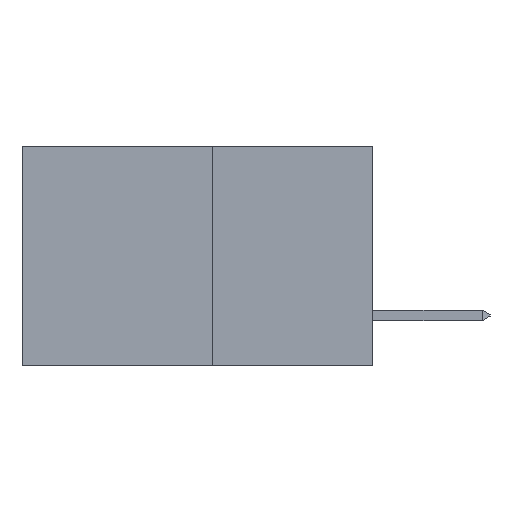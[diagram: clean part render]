
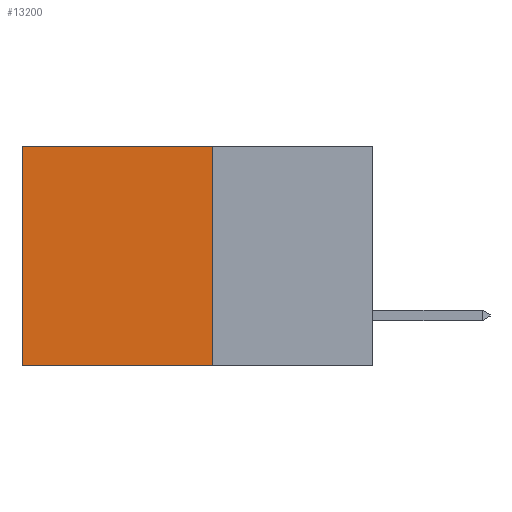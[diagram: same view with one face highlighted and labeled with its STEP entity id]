
A CAD part, left-side view. The second image highlights one B-rep face of the part: STEP entity #13200.
In plain terms, the highlighted planar face has unit normal (-1, 0, 0).
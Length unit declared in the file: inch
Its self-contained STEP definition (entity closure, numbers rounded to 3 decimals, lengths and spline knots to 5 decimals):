
#7 = DIRECTION ( 'NONE',  ( 0., 1., 0. ) ) ;
#88 = ORIENTED_EDGE ( 'NONE', *, *, #18496, .T. ) ;
#1582 = DIRECTION ( 'NONE',  ( 0., 0., -1. ) ) ;
#2198 = DIRECTION ( 'NONE',  ( 0., 0., -1. ) ) ;
#2292 = ORIENTED_EDGE ( 'NONE', *, *, #22013, .T. ) ;
#4181 = VERTEX_POINT ( 'NONE', #13359 ) ;
#4532 = CARTESIAN_POINT ( 'NONE',  ( 0.277, 0.27, -0.37 ) ) ;
#4536 = CARTESIAN_POINT ( 'NONE',  ( 0.277, 0.59, -0.37 ) ) ;
#6033 = LINE ( 'NONE', #4536, #24186 ) ;
#7980 = VECTOR ( 'NONE', #15490, 39.37008 ) ;
#8729 = LINE ( 'NONE', #22567, #7980 ) ;
#9309 = PLANE ( 'NONE',  #23987 ) ;
#9402 = CARTESIAN_POINT ( 'NONE',  ( 0.277, 0.59, -0.37 ) ) ;
#9446 = VERTEX_POINT ( 'NONE', #9402 ) ;
#10930 = ORIENTED_EDGE ( 'NONE', *, *, #21144, .F. ) ;
#13200 = ADVANCED_FACE ( 'NONE', ( #29827 ), #9309, .F. ) ;
#13251 = EDGE_CURVE ( 'NONE', #4181, #9446, #15998, .T. ) ;
#13359 = CARTESIAN_POINT ( 'NONE',  ( 0.277, 0.27, -0.37 ) ) ;
#13468 = VERTEX_POINT ( 'NONE', #26701 ) ;
#14346 = CARTESIAN_POINT ( 'NONE',  ( 0.277, 0.59, 0. ) ) ;
#15490 = DIRECTION ( 'NONE',  ( 0., 1., 0. ) ) ;
#15998 = LINE ( 'NONE', #28307, #21582 ) ;
#16497 = DIRECTION ( 'NONE',  ( 1., 0., 0. ) ) ;
#16927 = DIRECTION ( 'NONE',  ( 0., 0., -1. ) ) ;
#18496 = EDGE_CURVE ( 'NONE', #13468, #24908, #8729, .T. ) ;
#20213 = VECTOR ( 'NONE', #1582, 39.37008 ) ;
#20827 = EDGE_LOOP ( 'NONE', ( #2292, #29924, #10930, #88 ) ) ;
#20970 = LINE ( 'NONE', #29807, #20213 ) ;
#21144 = EDGE_CURVE ( 'NONE', #13468, #4181, #20970, .T. ) ;
#21582 = VECTOR ( 'NONE', #7, 39.37008 ) ;
#22013 = EDGE_CURVE ( 'NONE', #24908, #9446, #6033, .T. ) ;
#22567 = CARTESIAN_POINT ( 'NONE',  ( 0.277, 0.27, 0. ) ) ;
#23987 = AXIS2_PLACEMENT_3D ( 'NONE', #4532, #16497, #2198 ) ;
#24186 = VECTOR ( 'NONE', #16927, 39.37008 ) ;
#24908 = VERTEX_POINT ( 'NONE', #14346 ) ;
#26701 = CARTESIAN_POINT ( 'NONE',  ( 0.277, 0.27, 0. ) ) ;
#28307 = CARTESIAN_POINT ( 'NONE',  ( 0.277, 0.27, -0.37 ) ) ;
#29807 = CARTESIAN_POINT ( 'NONE',  ( 0.277, 0.27, -0.37 ) ) ;
#29827 = FACE_OUTER_BOUND ( 'NONE', #20827, .T. ) ;
#29924 = ORIENTED_EDGE ( 'NONE', *, *, #13251, .F. ) ;
